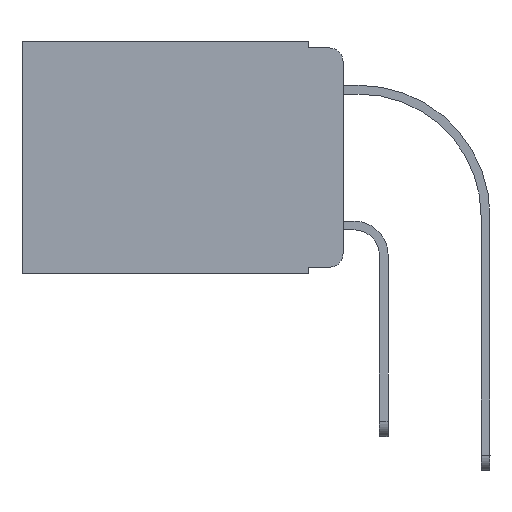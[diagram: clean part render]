
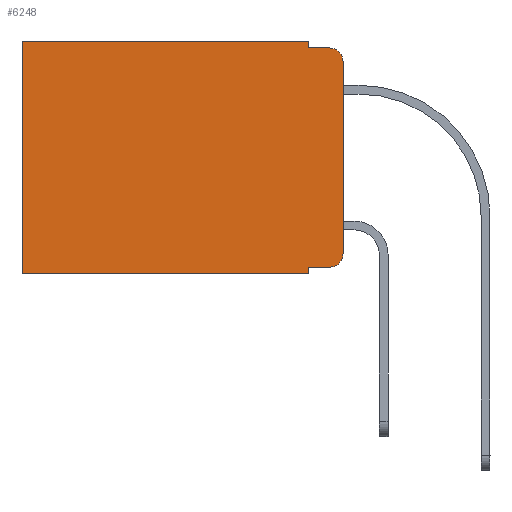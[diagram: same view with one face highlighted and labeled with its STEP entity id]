
A CAD part, left-side view. The second image highlights one B-rep face of the part: STEP entity #6248.
In plain terms, the highlighted planar face has unit normal (-1, 0, 0).
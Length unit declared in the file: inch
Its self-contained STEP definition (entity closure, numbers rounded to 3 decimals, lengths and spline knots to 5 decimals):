
#187 = EDGE_CURVE ( 'NONE', #14774, #15467, #17385, .T. ) ;
#583 = CARTESIAN_POINT ( 'NONE',  ( 0.298, 0.051, 0. ) ) ;
#778 = CARTESIAN_POINT ( 'NONE',  ( 0.298, 0., -0.03 ) ) ;
#982 = VECTOR ( 'NONE', #2053, 39.37008 ) ;
#1139 = CARTESIAN_POINT ( 'NONE',  ( 0.298, 0., -0.313 ) ) ;
#1403 = VECTOR ( 'NONE', #8692, 39.37008 ) ;
#1856 = VERTEX_POINT ( 'NONE', #2840 ) ;
#1873 = DIRECTION ( 'NONE',  ( 0., 0., -1. ) ) ;
#2053 = DIRECTION ( 'NONE',  ( 0., 0., -1. ) ) ;
#2340 = ORIENTED_EDGE ( 'NONE', *, *, #187, .T. ) ;
#2390 = EDGE_CURVE ( 'NONE', #19821, #7119, #3648, .T. ) ;
#2467 = CARTESIAN_POINT ( 'NONE',  ( 0.298, 0.051, -0.01 ) ) ;
#2668 = ORIENTED_EDGE ( 'NONE', *, *, #16023, .F. ) ;
#2840 = CARTESIAN_POINT ( 'NONE',  ( 0.298, 0.051, -0.343 ) ) ;
#2963 = CARTESIAN_POINT ( 'NONE',  ( 0.298, 0.051, 0. ) ) ;
#3301 = LINE ( 'NONE', #6054, #7607 ) ;
#3308 = ORIENTED_EDGE ( 'NONE', *, *, #25595, .T. ) ;
#3426 = AXIS2_PLACEMENT_3D ( 'NONE', #14840, #10191, #5262 ) ;
#3648 = CIRCLE ( 'NONE', #9146, 0.02 ) ;
#4809 = VECTOR ( 'NONE', #11868, 39.37008 ) ;
#5222 = VECTOR ( 'NONE', #6763, 39.37008 ) ;
#5262 = DIRECTION ( 'NONE',  ( 0., 0., -1. ) ) ;
#5470 = AXIS2_PLACEMENT_3D ( 'NONE', #15969, #5858, #22111 ) ;
#5637 = CARTESIAN_POINT ( 'NONE',  ( 0.298, 0.051, 0. ) ) ;
#5858 = DIRECTION ( 'NONE',  ( 1., 0., 0. ) ) ;
#6054 = CARTESIAN_POINT ( 'NONE',  ( 0.298, 0., -0.343 ) ) ;
#6089 = VECTOR ( 'NONE', #8673, 39.37008 ) ;
#6243 = CARTESIAN_POINT ( 'NONE',  ( 0.298, 0.051, -0.333 ) ) ;
#6248 = ADVANCED_FACE ( 'NONE', ( #19990 ), #26102, .F. ) ;
#6558 = LINE ( 'NONE', #583, #6089 ) ;
#6634 = VERTEX_POINT ( 'NONE', #15804 ) ;
#6763 = DIRECTION ( 'NONE',  ( 0., -1., 0. ) ) ;
#7072 = ORIENTED_EDGE ( 'NONE', *, *, #12892, .T. ) ;
#7119 = VERTEX_POINT ( 'NONE', #1139 ) ;
#7150 = EDGE_LOOP ( 'NONE', ( #14743, #14428, #16617, #2668, #2340, #3308, #17981, #14818, #7072, #13325 ) ) ;
#7607 = VECTOR ( 'NONE', #16164, 39.37008 ) ;
#7837 = LINE ( 'NONE', #25956, #14492 ) ;
#8620 = CARTESIAN_POINT ( 'NONE',  ( 0.298, 0.051, -0.333 ) ) ;
#8673 = DIRECTION ( 'NONE',  ( 0., 0., -1. ) ) ;
#8692 = DIRECTION ( 'NONE',  ( 0., -1., 0. ) ) ;
#9146 = AXIS2_PLACEMENT_3D ( 'NONE', #11559, #19704, #1873 ) ;
#10191 = DIRECTION ( 'NONE',  ( -1., 0., 0. ) ) ;
#10910 = CARTESIAN_POINT ( 'NONE',  ( 0.298, 0.02, -0.01 ) ) ;
#11474 = VERTEX_POINT ( 'NONE', #778 ) ;
#11487 = CIRCLE ( 'NONE', #3426, 0.02 ) ;
#11559 = CARTESIAN_POINT ( 'NONE',  ( 0.298, 0.02, -0.313 ) ) ;
#11602 = CARTESIAN_POINT ( 'NONE',  ( 0.298, 0., 0. ) ) ;
#11868 = DIRECTION ( 'NONE',  ( 0., 0., -1. ) ) ;
#11968 = CARTESIAN_POINT ( 'NONE',  ( 0.298, 0.051, -0.01 ) ) ;
#12714 = EDGE_CURVE ( 'NONE', #11474, #7119, #14351, .T. ) ;
#12892 = EDGE_CURVE ( 'NONE', #20164, #19821, #16752, .T. ) ;
#13325 = ORIENTED_EDGE ( 'NONE', *, *, #2390, .T. ) ;
#13698 = EDGE_CURVE ( 'NONE', #18717, #18549, #20696, .T. ) ;
#14351 = LINE ( 'NONE', #11602, #4809 ) ;
#14428 = ORIENTED_EDGE ( 'NONE', *, *, #17736, .T. ) ;
#14492 = VECTOR ( 'NONE', #20239, 39.37008 ) ;
#14743 = ORIENTED_EDGE ( 'NONE', *, *, #12714, .F. ) ;
#14774 = VERTEX_POINT ( 'NONE', #2963 ) ;
#14818 = ORIENTED_EDGE ( 'NONE', *, *, #15820, .F. ) ;
#14840 = CARTESIAN_POINT ( 'NONE',  ( 0.298, 0.02, -0.03 ) ) ;
#15467 = VERTEX_POINT ( 'NONE', #25789 ) ;
#15804 = CARTESIAN_POINT ( 'NONE',  ( 0.298, 0.473, -0.343 ) ) ;
#15820 = EDGE_CURVE ( 'NONE', #20164, #1856, #23873, .T. ) ;
#15969 = CARTESIAN_POINT ( 'NONE',  ( 0.298, 0., 0. ) ) ;
#16023 = EDGE_CURVE ( 'NONE', #14774, #18717, #6558, .T. ) ;
#16164 = DIRECTION ( 'NONE',  ( 0., 1., 0. ) ) ;
#16243 = VECTOR ( 'NONE', #21268, 39.37008 ) ;
#16617 = ORIENTED_EDGE ( 'NONE', *, *, #13698, .F. ) ;
#16752 = LINE ( 'NONE', #8620, #5222 ) ;
#17385 = LINE ( 'NONE', #25504, #16243 ) ;
#17736 = EDGE_CURVE ( 'NONE', #11474, #18549, #11487, .T. ) ;
#17981 = ORIENTED_EDGE ( 'NONE', *, *, #19198, .F. ) ;
#18549 = VERTEX_POINT ( 'NONE', #10910 ) ;
#18717 = VERTEX_POINT ( 'NONE', #11968 ) ;
#19198 = EDGE_CURVE ( 'NONE', #1856, #6634, #3301, .T. ) ;
#19704 = DIRECTION ( 'NONE',  ( -1., 0., 0. ) ) ;
#19821 = VERTEX_POINT ( 'NONE', #22531 ) ;
#19990 = FACE_OUTER_BOUND ( 'NONE', #7150, .T. ) ;
#20164 = VERTEX_POINT ( 'NONE', #6243 ) ;
#20239 = DIRECTION ( 'NONE',  ( 0., 0., -1. ) ) ;
#20696 = LINE ( 'NONE', #2467, #1403 ) ;
#21268 = DIRECTION ( 'NONE',  ( 0., 1., 0. ) ) ;
#22111 = DIRECTION ( 'NONE',  ( 0., 0., -1. ) ) ;
#22531 = CARTESIAN_POINT ( 'NONE',  ( 0.298, 0.02, -0.333 ) ) ;
#23873 = LINE ( 'NONE', #5637, #982 ) ;
#25504 = CARTESIAN_POINT ( 'NONE',  ( 0.298, 0., 0. ) ) ;
#25595 = EDGE_CURVE ( 'NONE', #15467, #6634, #7837, .T. ) ;
#25789 = CARTESIAN_POINT ( 'NONE',  ( 0.298, 0.473, 0. ) ) ;
#25956 = CARTESIAN_POINT ( 'NONE',  ( 0.298, 0.473, 0. ) ) ;
#26102 = PLANE ( 'NONE',  #5470 ) ;
